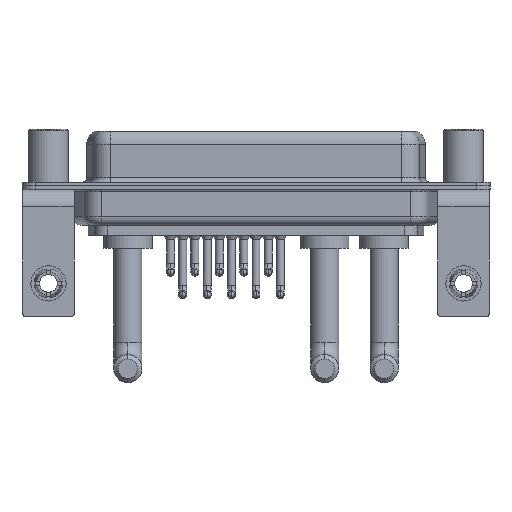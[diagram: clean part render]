
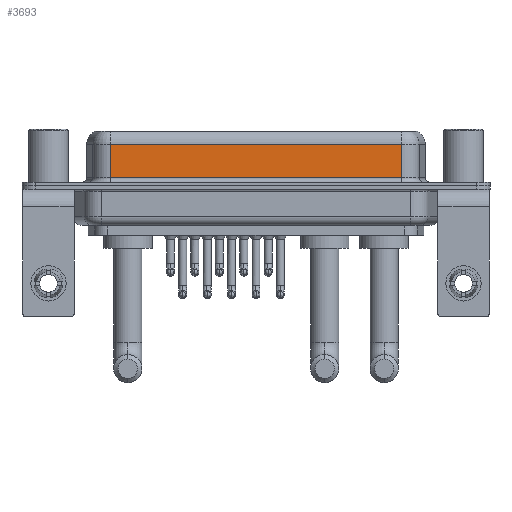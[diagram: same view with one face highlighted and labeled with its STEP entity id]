
A CAD part, front view. The second image highlights one B-rep face of the part: STEP entity #3693.
In plain terms, the highlighted planar face has unit normal (0, -1, 0).
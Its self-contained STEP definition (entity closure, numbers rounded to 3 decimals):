
#2161 = EDGE_CURVE ( 'NONE', #4646, #2969, #18055, .T. ) ;
#2969 = VERTEX_POINT ( 'NONE', #4153 ) ;
#3514 = ORIENTED_EDGE ( 'NONE', *, *, #14847, .F. ) ;
#3693 = ADVANCED_FACE ( 'NONE', ( #12083 ), #20993, .F. ) ;
#4153 = CARTESIAN_POINT ( 'NONE',  ( 40.037, -3.95, 0.9 ) ) ;
#4390 = ORIENTED_EDGE ( 'NONE', *, *, #21841, .T. ) ;
#4646 = VERTEX_POINT ( 'NONE', #19334 ) ;
#4927 = EDGE_CURVE ( 'NONE', #22508, #8641, #13040, .T. ) ;
#5430 = DIRECTION ( 'NONE',  ( 0., 0., -1. ) ) ;
#5607 = CARTESIAN_POINT ( 'NONE',  ( 40.037, -3.95, 0.9 ) ) ;
#6591 = CARTESIAN_POINT ( 'NONE',  ( 40.037, -3.95, 6.4 ) ) ;
#7548 = DIRECTION ( 'NONE',  ( 1., 0., 0. ) ) ;
#7777 = LINE ( 'NONE', #15938, #7787 ) ;
#7787 = VECTOR ( 'NONE', #5430, 1000. ) ;
#7954 = LINE ( 'NONE', #6591, #10148 ) ;
#8641 = VERTEX_POINT ( 'NONE', #19754 ) ;
#8774 = DIRECTION ( 'NONE',  ( 0., 0., 1. ) ) ;
#9485 = VECTOR ( 'NONE', #7548, 1000. ) ;
#10148 = VECTOR ( 'NONE', #13561, 1000. ) ;
#11540 = DIRECTION ( 'NONE',  ( -1., 0., 0. ) ) ;
#12083 = FACE_OUTER_BOUND ( 'NONE', #15781, .T. ) ;
#13040 = LINE ( 'NONE', #20231, #14312 ) ;
#13561 = DIRECTION ( 'NONE',  ( 0., 0., -1. ) ) ;
#14312 = VECTOR ( 'NONE', #11540, 1000. ) ;
#14847 = EDGE_CURVE ( 'NONE', #22508, #2969, #7954, .T. ) ;
#15781 = EDGE_LOOP ( 'NONE', ( #3514, #15891, #4390, #17341 ) ) ;
#15891 = ORIENTED_EDGE ( 'NONE', *, *, #4927, .T. ) ;
#15938 = CARTESIAN_POINT ( 'NONE',  ( 7.013, -3.95, 6.4 ) ) ;
#16074 = DIRECTION ( 'NONE',  ( 0., 1., 0. ) ) ;
#17341 = ORIENTED_EDGE ( 'NONE', *, *, #2161, .T. ) ;
#17680 = CARTESIAN_POINT ( 'NONE',  ( 40.037, -3.95, 4.65 ) ) ;
#17782 = CARTESIAN_POINT ( 'NONE',  ( 40.037, -3.95, 6.4 ) ) ;
#18055 = LINE ( 'NONE', #5607, #9485 ) ;
#19334 = CARTESIAN_POINT ( 'NONE',  ( 7.013, -3.95, 0.9 ) ) ;
#19754 = CARTESIAN_POINT ( 'NONE',  ( 7.013, -3.95, 4.65 ) ) ;
#20231 = CARTESIAN_POINT ( 'NONE',  ( 40.037, -3.95, 4.65 ) ) ;
#20993 = PLANE ( 'NONE',  #22260 ) ;
#21841 = EDGE_CURVE ( 'NONE', #8641, #4646, #7777, .T. ) ;
#22260 = AXIS2_PLACEMENT_3D ( 'NONE', #17782, #16074, #8774 ) ;
#22508 = VERTEX_POINT ( 'NONE', #17680 ) ;
